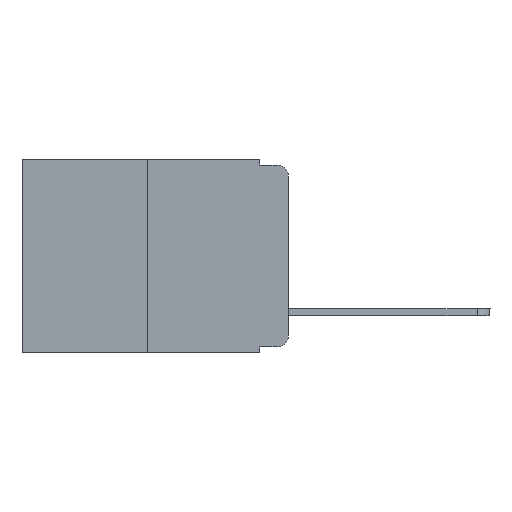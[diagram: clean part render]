
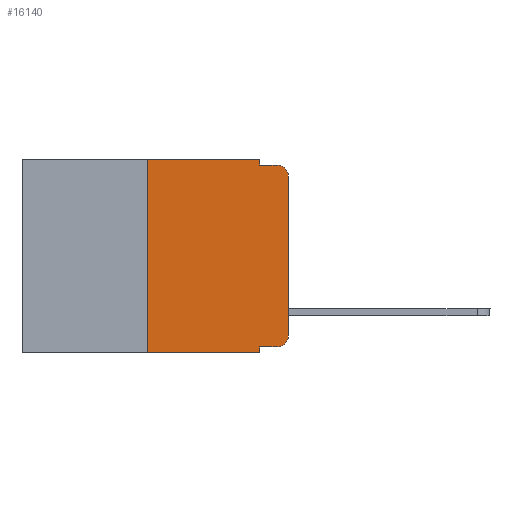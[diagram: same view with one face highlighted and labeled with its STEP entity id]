
A CAD part, left-side view. The second image highlights one B-rep face of the part: STEP entity #16140.
In plain terms, the highlighted planar face has unit normal (-1, 0, 0).
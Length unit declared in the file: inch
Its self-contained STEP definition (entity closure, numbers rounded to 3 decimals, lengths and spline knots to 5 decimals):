
#594 = ORIENTED_EDGE ( 'NONE', *, *, #15966, .F. ) ;
#1143 = CARTESIAN_POINT ( 'NONE',  ( 0., 0., -0.03 ) ) ;
#1208 = EDGE_LOOP ( 'NONE', ( #18026, #6817, #16181, #594, #16614, #10233, #5410, #1828, #3354, #5004 ) ) ;
#1559 = LINE ( 'NONE', #14194, #9922 ) ;
#1587 = VERTEX_POINT ( 'NONE', #1143 ) ;
#1828 = ORIENTED_EDGE ( 'NONE', *, *, #9771, .F. ) ;
#1956 = CARTESIAN_POINT ( 'NONE',  ( 0., 0.051, 0. ) ) ;
#2480 = CARTESIAN_POINT ( 'NONE',  ( 0., 0.25, 0. ) ) ;
#2505 = EDGE_CURVE ( 'NONE', #16363, #17452, #9758, .T. ) ;
#2575 = CARTESIAN_POINT ( 'NONE',  ( 0., 0.051, 0. ) ) ;
#2599 = DIRECTION ( 'NONE',  ( 0., -1., 0. ) ) ;
#2844 = VERTEX_POINT ( 'NONE', #10833 ) ;
#2874 = LINE ( 'NONE', #8622, #13222 ) ;
#3142 = VERTEX_POINT ( 'NONE', #17575 ) ;
#3354 = ORIENTED_EDGE ( 'NONE', *, *, #2505, .T. ) ;
#3874 = CARTESIAN_POINT ( 'NONE',  ( 0., 0.02, -0.333 ) ) ;
#4024 = EDGE_CURVE ( 'NONE', #12614, #16132, #6324, .T. ) ;
#4125 = EDGE_CURVE ( 'NONE', #5674, #1587, #13709, .T. ) ;
#4366 = VERTEX_POINT ( 'NONE', #7412 ) ;
#5004 = ORIENTED_EDGE ( 'NONE', *, *, #9513, .T. ) ;
#5197 = CIRCLE ( 'NONE', #13791, 0.02 ) ;
#5283 = DIRECTION ( 'NONE',  ( 0., 0., 1. ) ) ;
#5410 = ORIENTED_EDGE ( 'NONE', *, *, #14118, .T. ) ;
#5476 = AXIS2_PLACEMENT_3D ( 'NONE', #15008, #8138, #12056 ) ;
#5671 = CARTESIAN_POINT ( 'NONE',  ( 0., 0.02, -0.313 ) ) ;
#5674 = VERTEX_POINT ( 'NONE', #12216 ) ;
#5952 = DIRECTION ( 'NONE',  ( 0., -1., 0. ) ) ;
#6057 = VECTOR ( 'NONE', #5283, 39.37008 ) ;
#6248 = CARTESIAN_POINT ( 'NONE',  ( 0., 0.25, -0.343 ) ) ;
#6324 = LINE ( 'NONE', #10584, #11080 ) ;
#6720 = CARTESIAN_POINT ( 'NONE',  ( 0., 0.473, 0. ) ) ;
#6817 = ORIENTED_EDGE ( 'NONE', *, *, #13185, .T. ) ;
#6983 = VECTOR ( 'NONE', #16576, 39.37008 ) ;
#7388 = AXIS2_PLACEMENT_3D ( 'NONE', #15384, #18062, #12228 ) ;
#7412 = CARTESIAN_POINT ( 'NONE',  ( 0., 0.051, -0.343 ) ) ;
#7601 = VECTOR ( 'NONE', #2599, 39.37008 ) ;
#7689 = DIRECTION ( 'NONE',  ( 0., 0., -1. ) ) ;
#8138 = DIRECTION ( 'NONE',  ( -1., 0., 0. ) ) ;
#8422 = FACE_OUTER_BOUND ( 'NONE', #1208, .T. ) ;
#8622 = CARTESIAN_POINT ( 'NONE',  ( 0., 0.051, -0.01 ) ) ;
#9430 = EDGE_CURVE ( 'NONE', #15393, #3142, #2874, .T. ) ;
#9513 = EDGE_CURVE ( 'NONE', #17452, #5674, #5197, .T. ) ;
#9528 = LINE ( 'NONE', #2575, #6983 ) ;
#9697 = LINE ( 'NONE', #6720, #13769 ) ;
#9758 = LINE ( 'NONE', #16886, #7601 ) ;
#9771 = EDGE_CURVE ( 'NONE', #16363, #4366, #9528, .T. ) ;
#9922 = VECTOR ( 'NONE', #12531, 39.37008 ) ;
#9982 = DIRECTION ( 'NONE',  ( 0., -1., 0. ) ) ;
#10233 = ORIENTED_EDGE ( 'NONE', *, *, #4024, .F. ) ;
#10584 = CARTESIAN_POINT ( 'NONE',  ( 0., 0.25, 0. ) ) ;
#10761 = CIRCLE ( 'NONE', #5476, 0.02 ) ;
#10833 = CARTESIAN_POINT ( 'NONE',  ( 0., 0.051, 0. ) ) ;
#11080 = VECTOR ( 'NONE', #12233, 39.37008 ) ;
#11737 = CARTESIAN_POINT ( 'NONE',  ( 0., 0.051, -0.01 ) ) ;
#12056 = DIRECTION ( 'NONE',  ( 0., 0., -1. ) ) ;
#12216 = CARTESIAN_POINT ( 'NONE',  ( 0., 0., -0.313 ) ) ;
#12228 = DIRECTION ( 'NONE',  ( 0., 0., -1. ) ) ;
#12233 = DIRECTION ( 'NONE',  ( 0., 0., 1. ) ) ;
#12531 = DIRECTION ( 'NONE',  ( 0., -1., 0. ) ) ;
#12614 = VERTEX_POINT ( 'NONE', #6248 ) ;
#13185 = EDGE_CURVE ( 'NONE', #1587, #3142, #10761, .T. ) ;
#13222 = VECTOR ( 'NONE', #5952, 39.37008 ) ;
#13709 = LINE ( 'NONE', #17974, #6057 ) ;
#13769 = VECTOR ( 'NONE', #9982, 39.37008 ) ;
#13791 = AXIS2_PLACEMENT_3D ( 'NONE', #5671, #16964, #14192 ) ;
#14093 = PLANE ( 'NONE',  #7388 ) ;
#14115 = VECTOR ( 'NONE', #7689, 39.37008 ) ;
#14118 = EDGE_CURVE ( 'NONE', #12614, #4366, #1559, .T. ) ;
#14192 = DIRECTION ( 'NONE',  ( 0., 0., -1. ) ) ;
#14194 = CARTESIAN_POINT ( 'NONE',  ( 0., 0.473, -0.343 ) ) ;
#14898 = CARTESIAN_POINT ( 'NONE',  ( 0., 0.051, -0.333 ) ) ;
#15008 = CARTESIAN_POINT ( 'NONE',  ( 0., 0.02, -0.03 ) ) ;
#15335 = EDGE_CURVE ( 'NONE', #16132, #2844, #9697, .T. ) ;
#15384 = CARTESIAN_POINT ( 'NONE',  ( 0., 0.473, 0. ) ) ;
#15393 = VERTEX_POINT ( 'NONE', #11737 ) ;
#15966 = EDGE_CURVE ( 'NONE', #2844, #15393, #17704, .T. ) ;
#16132 = VERTEX_POINT ( 'NONE', #2480 ) ;
#16140 = ADVANCED_FACE ( 'NONE', ( #8422 ), #14093, .F. ) ;
#16181 = ORIENTED_EDGE ( 'NONE', *, *, #9430, .F. ) ;
#16363 = VERTEX_POINT ( 'NONE', #14898 ) ;
#16576 = DIRECTION ( 'NONE',  ( 0., 0., -1. ) ) ;
#16614 = ORIENTED_EDGE ( 'NONE', *, *, #15335, .F. ) ;
#16886 = CARTESIAN_POINT ( 'NONE',  ( 0., 0.051, -0.333 ) ) ;
#16964 = DIRECTION ( 'NONE',  ( -1., 0., 0. ) ) ;
#17452 = VERTEX_POINT ( 'NONE', #3874 ) ;
#17575 = CARTESIAN_POINT ( 'NONE',  ( 0., 0.02, -0.01 ) ) ;
#17704 = LINE ( 'NONE', #1956, #14115 ) ;
#17974 = CARTESIAN_POINT ( 'NONE',  ( 0., 0., 0. ) ) ;
#18026 = ORIENTED_EDGE ( 'NONE', *, *, #4125, .T. ) ;
#18062 = DIRECTION ( 'NONE',  ( 1., 0., 0. ) ) ;
